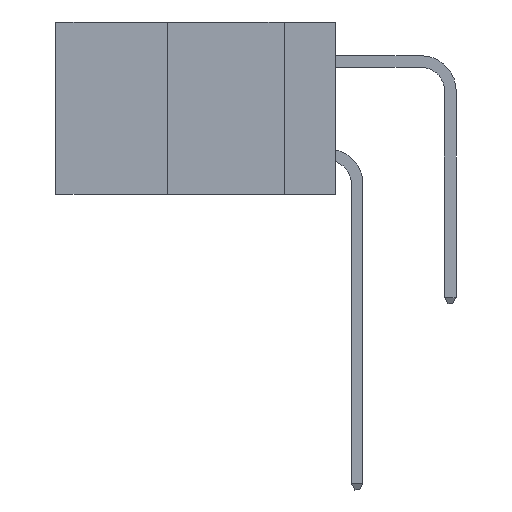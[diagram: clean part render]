
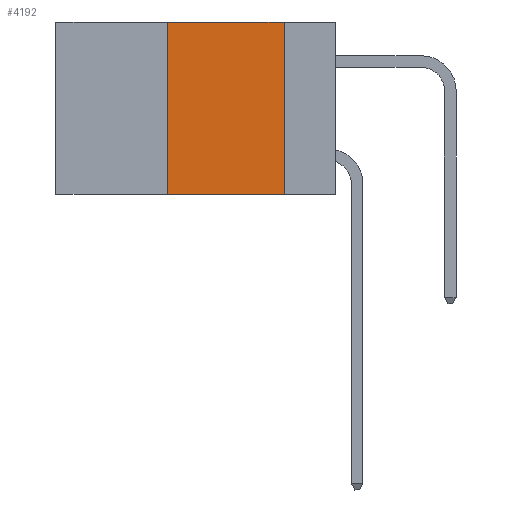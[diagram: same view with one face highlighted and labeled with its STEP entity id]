
A CAD part, left-side view. The second image highlights one B-rep face of the part: STEP entity #4192.
In plain terms, the highlighted planar face has unit normal (-1, 0, 0).
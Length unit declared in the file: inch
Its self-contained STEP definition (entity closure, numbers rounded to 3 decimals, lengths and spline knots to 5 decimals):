
#282 = VERTEX_POINT ( 'NONE', #11882 ) ;
#1061 = LINE ( 'NONE', #14345, #7666 ) ;
#1507 = FACE_OUTER_BOUND ( 'NONE', #3215, .T. ) ;
#2245 = ORIENTED_EDGE ( 'NONE', *, *, #9629, .T. ) ;
#2348 = ORIENTED_EDGE ( 'NONE', *, *, #13852, .F. ) ;
#2413 = AXIS2_PLACEMENT_3D ( 'NONE', #11549, #6074, #13618 ) ;
#3040 = LINE ( 'NONE', #11860, #5400 ) ;
#3215 = EDGE_LOOP ( 'NONE', ( #12611, #2348, #6330, #2245 ) ) ;
#3429 = LINE ( 'NONE', #7859, #6141 ) ;
#3765 = PLANE ( 'NONE',  #2413 ) ;
#3838 = VECTOR ( 'NONE', #11284, 39.37008 ) ;
#4083 = VERTEX_POINT ( 'NONE', #7057 ) ;
#4192 = ADVANCED_FACE ( 'NONE', ( #1507 ), #3765, .F. ) ;
#4222 = VERTEX_POINT ( 'NONE', #11593 ) ;
#4463 = CARTESIAN_POINT ( 'NONE',  ( 0., 0.36, 0. ) ) ;
#5400 = VECTOR ( 'NONE', #12884, 39.37008 ) ;
#5741 = CARTESIAN_POINT ( 'NONE',  ( 0., 0.36, 0. ) ) ;
#6027 = EDGE_CURVE ( 'NONE', #4083, #282, #1061, .T. ) ;
#6074 = DIRECTION ( 'NONE',  ( 1., 0., 0. ) ) ;
#6141 = VECTOR ( 'NONE', #14183, 39.37008 ) ;
#6330 = ORIENTED_EDGE ( 'NONE', *, *, #7383, .F. ) ;
#6919 = LINE ( 'NONE', #5741, #3838 ) ;
#7057 = CARTESIAN_POINT ( 'NONE',  ( 0., 0.11, 0. ) ) ;
#7383 = EDGE_CURVE ( 'NONE', #4222, #9179, #6919, .T. ) ;
#7666 = VECTOR ( 'NONE', #10177, 39.37008 ) ;
#7859 = CARTESIAN_POINT ( 'NONE',  ( 0., 0.6, 0. ) ) ;
#9179 = VERTEX_POINT ( 'NONE', #4463 ) ;
#9629 = EDGE_CURVE ( 'NONE', #4222, #282, #3040, .T. ) ;
#10177 = DIRECTION ( 'NONE',  ( 0., 0., -1. ) ) ;
#11284 = DIRECTION ( 'NONE',  ( 0., 0., 1. ) ) ;
#11549 = CARTESIAN_POINT ( 'NONE',  ( 0., 0.6, 0. ) ) ;
#11593 = CARTESIAN_POINT ( 'NONE',  ( 0., 0.36, -0.37 ) ) ;
#11860 = CARTESIAN_POINT ( 'NONE',  ( 0., 0.6, -0.37 ) ) ;
#11882 = CARTESIAN_POINT ( 'NONE',  ( 0., 0.11, -0.37 ) ) ;
#12611 = ORIENTED_EDGE ( 'NONE', *, *, #6027, .F. ) ;
#12884 = DIRECTION ( 'NONE',  ( 0., -1., 0. ) ) ;
#13618 = DIRECTION ( 'NONE',  ( 0., 0., -1. ) ) ;
#13852 = EDGE_CURVE ( 'NONE', #9179, #4083, #3429, .T. ) ;
#14183 = DIRECTION ( 'NONE',  ( 0., -1., 0. ) ) ;
#14345 = CARTESIAN_POINT ( 'NONE',  ( 0., 0.11, 0. ) ) ;
